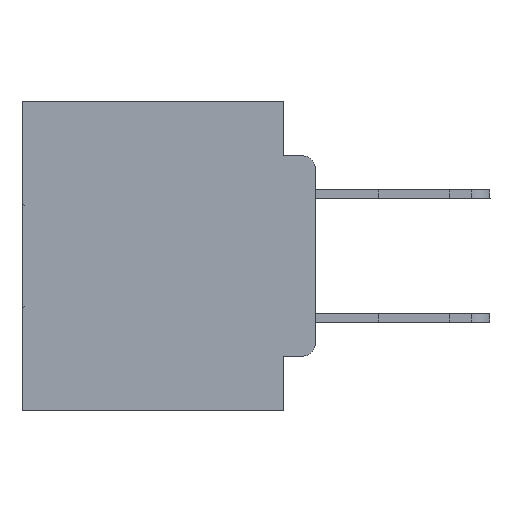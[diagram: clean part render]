
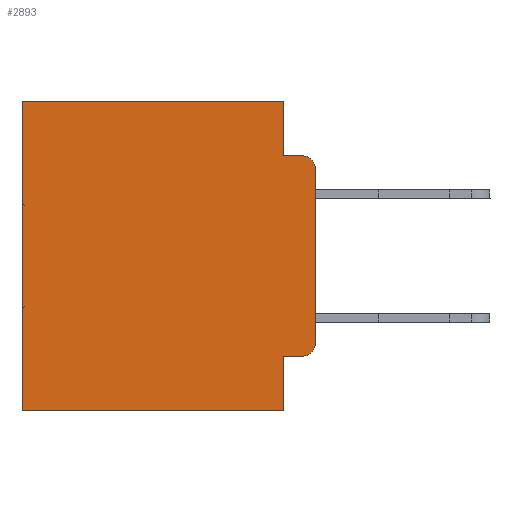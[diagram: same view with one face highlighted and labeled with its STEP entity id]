
A CAD part, left-side view. The second image highlights one B-rep face of the part: STEP entity #2893.
In plain terms, the highlighted planar face has unit normal (-1, 0, 0).
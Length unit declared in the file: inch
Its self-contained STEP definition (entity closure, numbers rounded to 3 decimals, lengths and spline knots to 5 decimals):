
#35 = DIRECTION ( 'NONE',  ( 0., 0., -1. ) ) ;
#231 = CARTESIAN_POINT ( 'NONE',  ( 0.298, 0., 0. ) ) ;
#826 = CARTESIAN_POINT ( 'NONE',  ( 0.298, 0.051, 0. ) ) ;
#954 = DIRECTION ( 'NONE',  ( 0., 0., -1. ) ) ;
#1388 = VECTOR ( 'NONE', #27991, 39.37008 ) ;
#1740 = CARTESIAN_POINT ( 'NONE',  ( 0.298, 0.02, -0.1085 ) ) ;
#2048 = CARTESIAN_POINT ( 'NONE',  ( 0.298, 0.051, 0. ) ) ;
#2703 = AXIS2_PLACEMENT_3D ( 'NONE', #231, #13231, #26135 ) ;
#2893 = ADVANCED_FACE ( 'NONE', ( #5630 ), #23286, .F. ) ;
#2926 = CARTESIAN_POINT ( 'NONE',  ( 0.298, 0.051, -0.0885 ) ) ;
#3140 = CARTESIAN_POINT ( 'NONE',  ( 0.298, 0.473, 0. ) ) ;
#3700 = EDGE_CURVE ( 'NONE', #21056, #31776, #31566, .T. ) ;
#3863 = VECTOR ( 'NONE', #8967, 39.37008 ) ;
#3925 = DIRECTION ( 'NONE',  ( 0., 0., -1. ) ) ;
#4013 = VECTOR ( 'NONE', #6024, 39.37008 ) ;
#5167 = VERTEX_POINT ( 'NONE', #19034 ) ;
#5483 = LINE ( 'NONE', #17953, #19073 ) ;
#5630 = FACE_OUTER_BOUND ( 'NONE', #22488, .T. ) ;
#5707 = ORIENTED_EDGE ( 'NONE', *, *, #28659, .T. ) ;
#5856 = LINE ( 'NONE', #29052, #4013 ) ;
#6024 = DIRECTION ( 'NONE',  ( 0., 1., 0. ) ) ;
#6037 = VERTEX_POINT ( 'NONE', #9760 ) ;
#6277 = LINE ( 'NONE', #11487, #3863 ) ;
#7040 = CARTESIAN_POINT ( 'NONE',  ( 0.298, 0.051, -0.0885 ) ) ;
#7136 = LINE ( 'NONE', #19923, #16889 ) ;
#7379 = ORIENTED_EDGE ( 'NONE', *, *, #20138, .T. ) ;
#7854 = EDGE_CURVE ( 'NONE', #15989, #31059, #28151, .T. ) ;
#8384 = CARTESIAN_POINT ( 'NONE',  ( 0.298, 0., -0.3915 ) ) ;
#8846 = AXIS2_PLACEMENT_3D ( 'NONE', #1740, #26960, #3925 ) ;
#8849 = DIRECTION ( 'NONE',  ( 0., 0., -1. ) ) ;
#8967 = DIRECTION ( 'NONE',  ( 0., -1., 0. ) ) ;
#9303 = EDGE_CURVE ( 'NONE', #6037, #13686, #26309, .T. ) ;
#9760 = CARTESIAN_POINT ( 'NONE',  ( 0.298, 0., -0.1085 ) ) ;
#10241 = DIRECTION ( 'NONE',  ( 0., 0., -1. ) ) ;
#11160 = VERTEX_POINT ( 'NONE', #17379 ) ;
#11487 = CARTESIAN_POINT ( 'NONE',  ( 0.298, 0.051, -0.4115 ) ) ;
#11704 = AXIS2_PLACEMENT_3D ( 'NONE', #14972, #12910, #10241 ) ;
#12910 = DIRECTION ( 'NONE',  ( -1., 0., 0. ) ) ;
#13231 = DIRECTION ( 'NONE',  ( 1., 0., 0. ) ) ;
#13300 = ORIENTED_EDGE ( 'NONE', *, *, #26043, .F. ) ;
#13347 = CARTESIAN_POINT ( 'NONE',  ( 0.298, 0.02, -0.0885 ) ) ;
#13637 = CARTESIAN_POINT ( 'NONE',  ( 0.298, 0.473, 0. ) ) ;
#13686 = VERTEX_POINT ( 'NONE', #8384 ) ;
#13750 = CARTESIAN_POINT ( 'NONE',  ( 0.298, 0., 0. ) ) ;
#14972 = CARTESIAN_POINT ( 'NONE',  ( 0.298, 0.02, -0.3915 ) ) ;
#15735 = VERTEX_POINT ( 'NONE', #826 ) ;
#15989 = VERTEX_POINT ( 'NONE', #7040 ) ;
#16645 = EDGE_CURVE ( 'NONE', #5167, #11160, #6277, .T. ) ;
#16889 = VECTOR ( 'NONE', #35, 39.37008 ) ;
#17266 = ORIENTED_EDGE ( 'NONE', *, *, #25459, .F. ) ;
#17379 = CARTESIAN_POINT ( 'NONE',  ( 0.298, 0.02, -0.4115 ) ) ;
#17953 = CARTESIAN_POINT ( 'NONE',  ( 0.298, 0., 0. ) ) ;
#18137 = CIRCLE ( 'NONE', #11704, 0.02 ) ;
#19034 = CARTESIAN_POINT ( 'NONE',  ( 0.298, 0.051, -0.4115 ) ) ;
#19073 = VECTOR ( 'NONE', #28173, 39.37008 ) ;
#19426 = VERTEX_POINT ( 'NONE', #32127 ) ;
#19923 = CARTESIAN_POINT ( 'NONE',  ( 0.298, 0.051, 0. ) ) ;
#19977 = CARTESIAN_POINT ( 'NONE',  ( 0.298, 0.473, -0.5 ) ) ;
#20138 = EDGE_CURVE ( 'NONE', #15735, #21056, #5483, .T. ) ;
#20251 = DIRECTION ( 'NONE',  ( 0., 0., -1. ) ) ;
#20330 = ORIENTED_EDGE ( 'NONE', *, *, #16645, .T. ) ;
#20406 = LINE ( 'NONE', #2048, #31575 ) ;
#21056 = VERTEX_POINT ( 'NONE', #13637 ) ;
#22488 = EDGE_LOOP ( 'NONE', ( #24396, #29594, #30328, #23314, #7379, #26715, #13300, #17266, #20330, #5707 ) ) ;
#23286 = PLANE ( 'NONE',  #2703 ) ;
#23314 = ORIENTED_EDGE ( 'NONE', *, *, #29577, .F. ) ;
#24396 = ORIENTED_EDGE ( 'NONE', *, *, #9303, .F. ) ;
#25337 = EDGE_CURVE ( 'NONE', #6037, #31059, #32431, .T. ) ;
#25459 = EDGE_CURVE ( 'NONE', #5167, #19426, #7136, .T. ) ;
#25961 = VECTOR ( 'NONE', #954, 39.37008 ) ;
#26043 = EDGE_CURVE ( 'NONE', #19426, #31776, #5856, .T. ) ;
#26135 = DIRECTION ( 'NONE',  ( 0., 0., -1. ) ) ;
#26309 = LINE ( 'NONE', #13750, #29228 ) ;
#26715 = ORIENTED_EDGE ( 'NONE', *, *, #3700, .T. ) ;
#26960 = DIRECTION ( 'NONE',  ( -1., 0., 0. ) ) ;
#27991 = DIRECTION ( 'NONE',  ( 0., -1., 0. ) ) ;
#28151 = LINE ( 'NONE', #2926, #1388 ) ;
#28173 = DIRECTION ( 'NONE',  ( 0., 1., 0. ) ) ;
#28659 = EDGE_CURVE ( 'NONE', #11160, #13686, #18137, .T. ) ;
#29052 = CARTESIAN_POINT ( 'NONE',  ( 0.298, 0., -0.5 ) ) ;
#29228 = VECTOR ( 'NONE', #8849, 39.37008 ) ;
#29577 = EDGE_CURVE ( 'NONE', #15735, #15989, #20406, .T. ) ;
#29594 = ORIENTED_EDGE ( 'NONE', *, *, #25337, .T. ) ;
#30328 = ORIENTED_EDGE ( 'NONE', *, *, #7854, .F. ) ;
#31059 = VERTEX_POINT ( 'NONE', #13347 ) ;
#31566 = LINE ( 'NONE', #3140, #25961 ) ;
#31575 = VECTOR ( 'NONE', #20251, 39.37008 ) ;
#31776 = VERTEX_POINT ( 'NONE', #19977 ) ;
#32127 = CARTESIAN_POINT ( 'NONE',  ( 0.298, 0.051, -0.5 ) ) ;
#32431 = CIRCLE ( 'NONE', #8846, 0.02 ) ;
